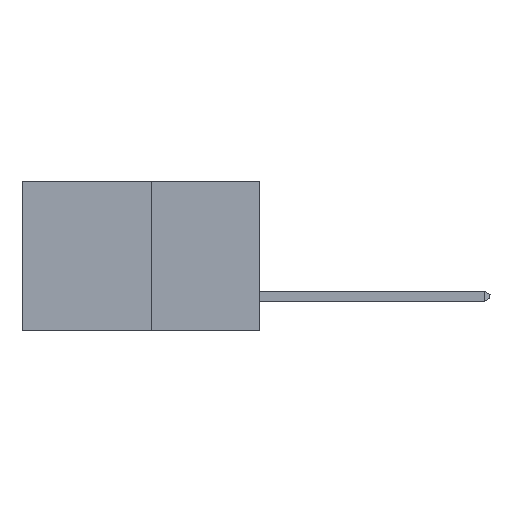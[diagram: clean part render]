
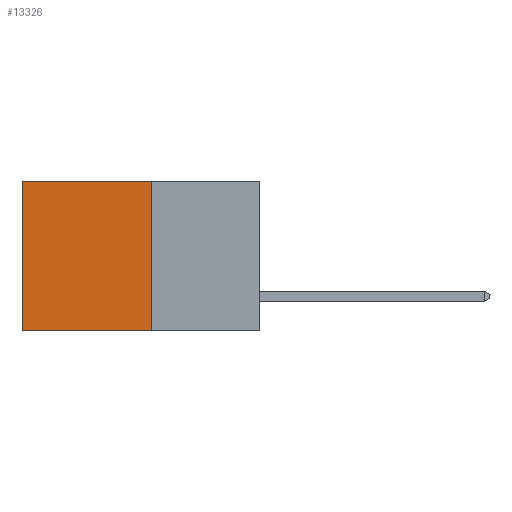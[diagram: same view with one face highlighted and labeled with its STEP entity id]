
A CAD part, left-side view. The second image highlights one B-rep face of the part: STEP entity #13326.
In plain terms, the highlighted planar face has unit normal (-1, 0, 0).
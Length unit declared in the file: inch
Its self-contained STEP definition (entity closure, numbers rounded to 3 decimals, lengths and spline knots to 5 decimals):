
#1051 = DIRECTION ( 'NONE',  ( 1., 0., 0. ) ) ;
#1771 = CARTESIAN_POINT ( 'NONE',  ( 0.277, 0.27, 0. ) ) ;
#2222 = EDGE_CURVE ( 'NONE', #3719, #10764, #11713, .T. ) ;
#3404 = CARTESIAN_POINT ( 'NONE',  ( 0.277, 0.59, -0.37 ) ) ;
#3451 = VERTEX_POINT ( 'NONE', #15446 ) ;
#3719 = VERTEX_POINT ( 'NONE', #13234 ) ;
#4311 = VERTEX_POINT ( 'NONE', #7395 ) ;
#4362 = LINE ( 'NONE', #3404, #7734 ) ;
#4552 = EDGE_LOOP ( 'NONE', ( #5477, #8520, #5845, #14937 ) ) ;
#4651 = CARTESIAN_POINT ( 'NONE',  ( 0.277, 0.27, -0.37 ) ) ;
#4949 = PLANE ( 'NONE',  #10820 ) ;
#5477 = ORIENTED_EDGE ( 'NONE', *, *, #15105, .T. ) ;
#5845 = ORIENTED_EDGE ( 'NONE', *, *, #2222, .F. ) ;
#6009 = VECTOR ( 'NONE', #9809, 39.37008 ) ;
#6426 = CARTESIAN_POINT ( 'NONE',  ( 0.277, 0.27, -0.37 ) ) ;
#6709 = LINE ( 'NONE', #6426, #6009 ) ;
#7395 = CARTESIAN_POINT ( 'NONE',  ( 0.277, 0.59, -0.37 ) ) ;
#7734 = VECTOR ( 'NONE', #9267, 39.37008 ) ;
#8318 = VECTOR ( 'NONE', #13756, 39.37008 ) ;
#8520 = ORIENTED_EDGE ( 'NONE', *, *, #10366, .F. ) ;
#8641 = LINE ( 'NONE', #1771, #14723 ) ;
#9267 = DIRECTION ( 'NONE',  ( 0., 0., -1. ) ) ;
#9558 = DIRECTION ( 'NONE',  ( 0., 0., -1. ) ) ;
#9809 = DIRECTION ( 'NONE',  ( 0., 1., 0. ) ) ;
#10166 = DIRECTION ( 'NONE',  ( 0., 1., 0. ) ) ;
#10366 = EDGE_CURVE ( 'NONE', #10764, #4311, #6709, .T. ) ;
#10764 = VERTEX_POINT ( 'NONE', #4651 ) ;
#10820 = AXIS2_PLACEMENT_3D ( 'NONE', #14118, #1051, #9558 ) ;
#10935 = FACE_OUTER_BOUND ( 'NONE', #4552, .T. ) ;
#11713 = LINE ( 'NONE', #12860, #8318 ) ;
#12209 = EDGE_CURVE ( 'NONE', #3719, #3451, #8641, .T. ) ;
#12860 = CARTESIAN_POINT ( 'NONE',  ( 0.277, 0.27, -0.37 ) ) ;
#13234 = CARTESIAN_POINT ( 'NONE',  ( 0.277, 0.27, 0. ) ) ;
#13326 = ADVANCED_FACE ( 'NONE', ( #10935 ), #4949, .F. ) ;
#13756 = DIRECTION ( 'NONE',  ( 0., 0., -1. ) ) ;
#14118 = CARTESIAN_POINT ( 'NONE',  ( 0.277, 0.27, -0.37 ) ) ;
#14723 = VECTOR ( 'NONE', #10166, 39.37008 ) ;
#14937 = ORIENTED_EDGE ( 'NONE', *, *, #12209, .T. ) ;
#15105 = EDGE_CURVE ( 'NONE', #3451, #4311, #4362, .T. ) ;
#15446 = CARTESIAN_POINT ( 'NONE',  ( 0.277, 0.59, 0. ) ) ;
